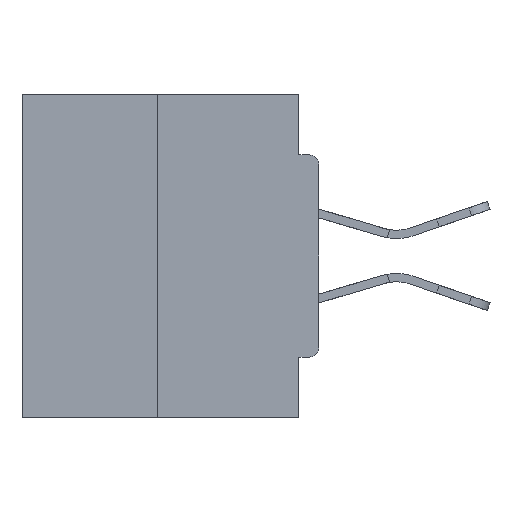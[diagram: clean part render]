
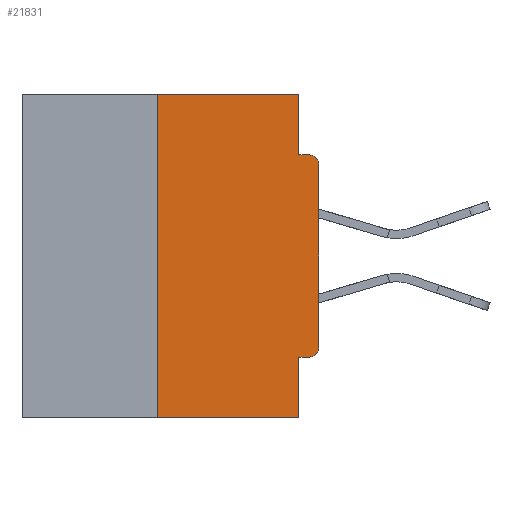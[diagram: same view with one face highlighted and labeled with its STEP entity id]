
A CAD part, left-side view. The second image highlights one B-rep face of the part: STEP entity #21831.
In plain terms, the highlighted planar face has unit normal (-1, 0, 0).
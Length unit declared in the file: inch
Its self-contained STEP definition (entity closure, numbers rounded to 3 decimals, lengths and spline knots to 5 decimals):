
#185 = FACE_OUTER_BOUND ( 'NONE', #6722, .T. ) ;
#407 = DIRECTION ( 'NONE',  ( 0., -1., 0. ) ) ;
#693 = ORIENTED_EDGE ( 'NONE', *, *, #19395, .F. ) ;
#1068 = VECTOR ( 'NONE', #16541, 39.37008 ) ;
#2412 = VERTEX_POINT ( 'NONE', #7264 ) ;
#3110 = CARTESIAN_POINT ( 'NONE',  ( 0., 0., 0. ) ) ;
#3287 = EDGE_CURVE ( 'NONE', #5216, #38723, #27872, .T. ) ;
#3437 = LINE ( 'NONE', #33070, #9464 ) ;
#3600 = ORIENTED_EDGE ( 'NONE', *, *, #27198, .T. ) ;
#3705 = DIRECTION ( 'NONE',  ( -1., 0., 0. ) ) ;
#3859 = CARTESIAN_POINT ( 'NONE',  ( 0., 0.015, -0.3915 ) ) ;
#4171 = CIRCLE ( 'NONE', #30943, 0.015 ) ;
#5216 = VERTEX_POINT ( 'NONE', #29387 ) ;
#5445 = CARTESIAN_POINT ( 'NONE',  ( 0., 0., -0.4065 ) ) ;
#5539 = CARTESIAN_POINT ( 'NONE',  ( 0., 0.031, 0. ) ) ;
#6001 = EDGE_CURVE ( 'NONE', #23755, #12041, #29805, .T. ) ;
#6201 = VECTOR ( 'NONE', #27636, 39.37008 ) ;
#6722 = EDGE_LOOP ( 'NONE', ( #36415, #34375, #37797, #22394, #20639, #3600, #40623, #9108, #24001, #693 ) ) ;
#7264 = CARTESIAN_POINT ( 'NONE',  ( 0., 0.031, -0.0935 ) ) ;
#7350 = CARTESIAN_POINT ( 'NONE',  ( 0., 0.031, -0.5 ) ) ;
#8633 = VECTOR ( 'NONE', #12862, 39.37008 ) ;
#9041 = DIRECTION ( 'NONE',  ( 1., 0., 0. ) ) ;
#9108 = ORIENTED_EDGE ( 'NONE', *, *, #19728, .T. ) ;
#9415 = DIRECTION ( 'NONE',  ( -1., 0., 0. ) ) ;
#9464 = VECTOR ( 'NONE', #23177, 39.37008 ) ;
#11058 = DIRECTION ( 'NONE',  ( 0., 0., -1. ) ) ;
#12041 = VERTEX_POINT ( 'NONE', #14153 ) ;
#12862 = DIRECTION ( 'NONE',  ( 0., 0., -1. ) ) ;
#14153 = CARTESIAN_POINT ( 'NONE',  ( 0., 0., -0.1085 ) ) ;
#14871 = EDGE_CURVE ( 'NONE', #19571, #28681, #38006, .T. ) ;
#15891 = EDGE_CURVE ( 'NONE', #2412, #37891, #3437, .T. ) ;
#16500 = DIRECTION ( 'NONE',  ( 0., 0., -1. ) ) ;
#16541 = DIRECTION ( 'NONE',  ( 0., 0., 1. ) ) ;
#16877 = VECTOR ( 'NONE', #407, 39.37008 ) ;
#18076 = DIRECTION ( 'NONE',  ( 0., -1., 0. ) ) ;
#19133 = DIRECTION ( 'NONE',  ( 0., 1., 0. ) ) ;
#19395 = EDGE_CURVE ( 'NONE', #28681, #2412, #44206, .T. ) ;
#19477 = PLANE ( 'NONE',  #28947 ) ;
#19571 = VERTEX_POINT ( 'NONE', #40463 ) ;
#19728 = EDGE_CURVE ( 'NONE', #12041, #37891, #4171, .T. ) ;
#20124 = CARTESIAN_POINT ( 'NONE',  ( 0., 0.015, -0.1085 ) ) ;
#20639 = ORIENTED_EDGE ( 'NONE', *, *, #3287, .F. ) ;
#21779 = CARTESIAN_POINT ( 'NONE',  ( 0., 0., -0.3915 ) ) ;
#21831 = ADVANCED_FACE ( 'NONE', ( #185 ), #19477, .F. ) ;
#22394 = ORIENTED_EDGE ( 'NONE', *, *, #35466, .F. ) ;
#23177 = DIRECTION ( 'NONE',  ( 0., -1., 0. ) ) ;
#23469 = CARTESIAN_POINT ( 'NONE',  ( 0., 0.015, -0.0935 ) ) ;
#23755 = VERTEX_POINT ( 'NONE', #21779 ) ;
#24001 = ORIENTED_EDGE ( 'NONE', *, *, #15891, .F. ) ;
#25728 = EDGE_CURVE ( 'NONE', #45193, #38198, #26172, .T. ) ;
#26172 = LINE ( 'NONE', #35882, #16877 ) ;
#26762 = VECTOR ( 'NONE', #19133, 39.37008 ) ;
#26870 = LINE ( 'NONE', #26938, #1068 ) ;
#26938 = CARTESIAN_POINT ( 'NONE',  ( 0., 0.25, 0. ) ) ;
#27198 = EDGE_CURVE ( 'NONE', #5216, #23755, #38475, .T. ) ;
#27369 = VECTOR ( 'NONE', #11058, 39.37008 ) ;
#27636 = DIRECTION ( 'NONE',  ( 0., 0., 1. ) ) ;
#27872 = LINE ( 'NONE', #5445, #26762 ) ;
#28190 = CARTESIAN_POINT ( 'NONE',  ( 0., 0.031, -0.4065 ) ) ;
#28681 = VERTEX_POINT ( 'NONE', #5539 ) ;
#28947 = AXIS2_PLACEMENT_3D ( 'NONE', #40240, #9041, #40562 ) ;
#29387 = CARTESIAN_POINT ( 'NONE',  ( 0., 0.015, -0.4065 ) ) ;
#29805 = LINE ( 'NONE', #3110, #6201 ) ;
#30564 = CARTESIAN_POINT ( 'NONE',  ( 0., 0.031, 0. ) ) ;
#30943 = AXIS2_PLACEMENT_3D ( 'NONE', #20124, #9415, #16500 ) ;
#33051 = EDGE_CURVE ( 'NONE', #45193, #19571, #26870, .T. ) ;
#33070 = CARTESIAN_POINT ( 'NONE',  ( 0., 0., -0.0935 ) ) ;
#33088 = VECTOR ( 'NONE', #18076, 39.37008 ) ;
#34375 = ORIENTED_EDGE ( 'NONE', *, *, #33051, .F. ) ;
#35466 = EDGE_CURVE ( 'NONE', #38723, #38198, #37686, .T. ) ;
#35882 = CARTESIAN_POINT ( 'NONE',  ( 0., 0.46, -0.5 ) ) ;
#36076 = AXIS2_PLACEMENT_3D ( 'NONE', #3859, #3705, #42745 ) ;
#36415 = ORIENTED_EDGE ( 'NONE', *, *, #14871, .F. ) ;
#37686 = LINE ( 'NONE', #7350, #27369 ) ;
#37797 = ORIENTED_EDGE ( 'NONE', *, *, #25728, .T. ) ;
#37891 = VERTEX_POINT ( 'NONE', #23469 ) ;
#37929 = CARTESIAN_POINT ( 'NONE',  ( 0., 0.46, 0. ) ) ;
#38006 = LINE ( 'NONE', #37929, #33088 ) ;
#38198 = VERTEX_POINT ( 'NONE', #38706 ) ;
#38475 = CIRCLE ( 'NONE', #36076, 0.015 ) ;
#38706 = CARTESIAN_POINT ( 'NONE',  ( 0., 0.031, -0.5 ) ) ;
#38723 = VERTEX_POINT ( 'NONE', #28190 ) ;
#39049 = CARTESIAN_POINT ( 'NONE',  ( 0., 0.25, -0.5 ) ) ;
#40240 = CARTESIAN_POINT ( 'NONE',  ( 0., 0.46, 0. ) ) ;
#40463 = CARTESIAN_POINT ( 'NONE',  ( 0., 0.25, 0. ) ) ;
#40562 = DIRECTION ( 'NONE',  ( 0., 0., -1. ) ) ;
#40623 = ORIENTED_EDGE ( 'NONE', *, *, #6001, .T. ) ;
#42745 = DIRECTION ( 'NONE',  ( 0., 0., -1. ) ) ;
#44206 = LINE ( 'NONE', #30564, #8633 ) ;
#45193 = VERTEX_POINT ( 'NONE', #39049 ) ;
